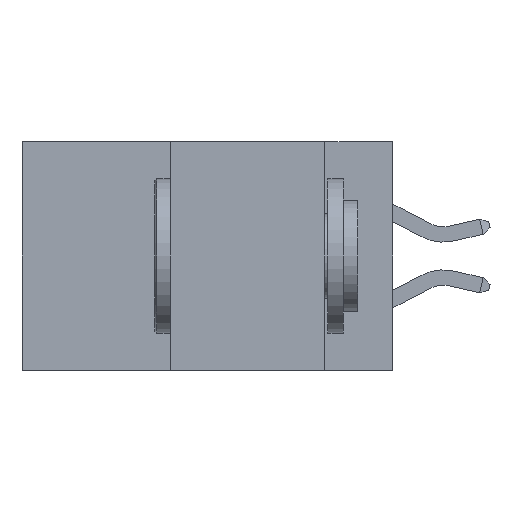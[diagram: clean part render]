
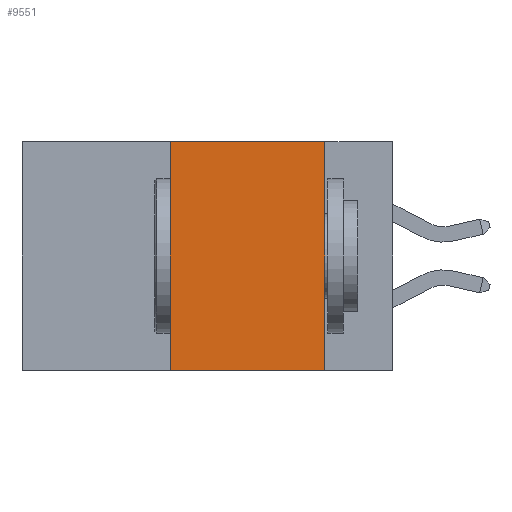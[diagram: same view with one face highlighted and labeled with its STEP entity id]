
A CAD part, left-side view. The second image highlights one B-rep face of the part: STEP entity #9551.
In plain terms, the highlighted planar face has unit normal (-1, 0, 0).
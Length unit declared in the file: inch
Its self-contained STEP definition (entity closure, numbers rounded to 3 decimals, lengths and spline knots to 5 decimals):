
#469 = LINE ( 'NONE', #7042, #8733 ) ;
#839 = EDGE_CURVE ( 'NONE', #9681, #4958, #8090, .T. ) ;
#1522 = CARTESIAN_POINT ( 'NONE',  ( 0., 0.11, 0. ) ) ;
#1663 = LINE ( 'NONE', #3753, #3417 ) ;
#2647 = CARTESIAN_POINT ( 'NONE',  ( 0., 0.36, -0.37 ) ) ;
#2743 = VERTEX_POINT ( 'NONE', #1522 ) ;
#3417 = VECTOR ( 'NONE', #8328, 39.37008 ) ;
#3447 = DIRECTION ( 'NONE',  ( 0., 0., -1. ) ) ;
#3449 = CARTESIAN_POINT ( 'NONE',  ( 0., 0.6, -0.37 ) ) ;
#3512 = DIRECTION ( 'NONE',  ( 0., 0., -1. ) ) ;
#3753 = CARTESIAN_POINT ( 'NONE',  ( 0., 0.36, 0. ) ) ;
#4221 = EDGE_CURVE ( 'NONE', #4324, #2743, #469, .T. ) ;
#4324 = VERTEX_POINT ( 'NONE', #5160 ) ;
#4723 = VECTOR ( 'NONE', #7978, 39.37008 ) ;
#4724 = PLANE ( 'NONE',  #7484 ) ;
#4958 = VERTEX_POINT ( 'NONE', #8436 ) ;
#5160 = CARTESIAN_POINT ( 'NONE',  ( 0., 0.36, 0. ) ) ;
#5165 = ORIENTED_EDGE ( 'NONE', *, *, #4221, .F. ) ;
#5493 = EDGE_CURVE ( 'NONE', #9681, #4324, #1663, .T. ) ;
#5495 = EDGE_LOOP ( 'NONE', ( #13595, #5165, #14038, #12573 ) ) ;
#5872 = CARTESIAN_POINT ( 'NONE',  ( 0., 0.6, 0. ) ) ;
#6788 = FACE_OUTER_BOUND ( 'NONE', #5495, .T. ) ;
#7042 = CARTESIAN_POINT ( 'NONE',  ( 0., 0.6, 0. ) ) ;
#7484 = AXIS2_PLACEMENT_3D ( 'NONE', #5872, #9268, #3512 ) ;
#7978 = DIRECTION ( 'NONE',  ( 0., -1., 0. ) ) ;
#8090 = LINE ( 'NONE', #3449, #4723 ) ;
#8263 = EDGE_CURVE ( 'NONE', #2743, #4958, #11921, .T. ) ;
#8270 = DIRECTION ( 'NONE',  ( 0., -1., 0. ) ) ;
#8328 = DIRECTION ( 'NONE',  ( 0., 0., 1. ) ) ;
#8436 = CARTESIAN_POINT ( 'NONE',  ( 0., 0.11, -0.37 ) ) ;
#8733 = VECTOR ( 'NONE', #8270, 39.37008 ) ;
#9268 = DIRECTION ( 'NONE',  ( 1., 0., 0. ) ) ;
#9551 = ADVANCED_FACE ( 'NONE', ( #6788 ), #4724, .F. ) ;
#9681 = VERTEX_POINT ( 'NONE', #2647 ) ;
#11921 = LINE ( 'NONE', #12468, #12591 ) ;
#12468 = CARTESIAN_POINT ( 'NONE',  ( 0., 0.11, 0. ) ) ;
#12573 = ORIENTED_EDGE ( 'NONE', *, *, #839, .T. ) ;
#12591 = VECTOR ( 'NONE', #3447, 39.37008 ) ;
#13595 = ORIENTED_EDGE ( 'NONE', *, *, #8263, .F. ) ;
#14038 = ORIENTED_EDGE ( 'NONE', *, *, #5493, .F. ) ;
